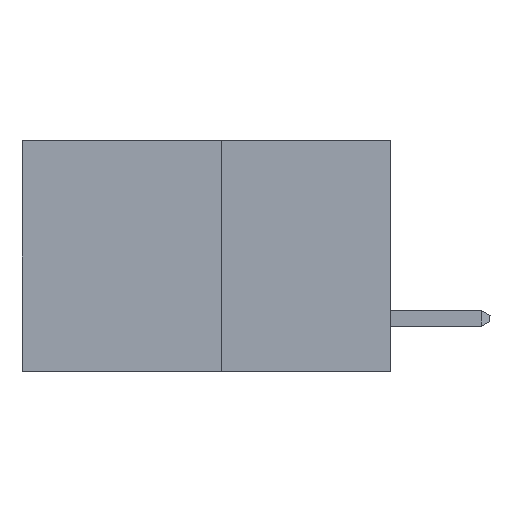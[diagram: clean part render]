
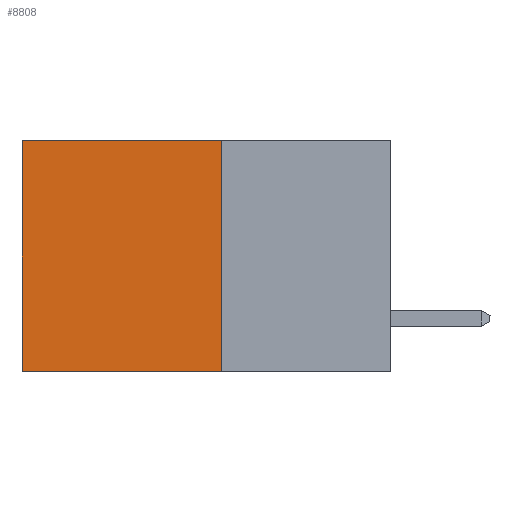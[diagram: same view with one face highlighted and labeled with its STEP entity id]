
A CAD part, left-side view. The second image highlights one B-rep face of the part: STEP entity #8808.
In plain terms, the highlighted planar face has unit normal (-1, 0, 0).
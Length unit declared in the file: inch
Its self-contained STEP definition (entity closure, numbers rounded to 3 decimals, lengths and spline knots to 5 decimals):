
#625 = VERTEX_POINT ( 'NONE', #13277 ) ;
#652 = EDGE_LOOP ( 'NONE', ( #5169, #15168, #2578, #5939 ) ) ;
#1002 = CARTESIAN_POINT ( 'NONE',  ( 0.277, 0.59, 0. ) ) ;
#1763 = CARTESIAN_POINT ( 'NONE',  ( 0.277, 0.27, -0.37 ) ) ;
#1943 = VERTEX_POINT ( 'NONE', #8669 ) ;
#2157 = EDGE_CURVE ( 'NONE', #6967, #1943, #5131, .T. ) ;
#2578 = ORIENTED_EDGE ( 'NONE', *, *, #9826, .F. ) ;
#4284 = LINE ( 'NONE', #13473, #10520 ) ;
#4394 = EDGE_CURVE ( 'NONE', #625, #14822, #4284, .T. ) ;
#4422 = DIRECTION ( 'NONE',  ( 0., 0., -1. ) ) ;
#4571 = CARTESIAN_POINT ( 'NONE',  ( 0.277, 0.27, -0.37 ) ) ;
#4724 = DIRECTION ( 'NONE',  ( 0., 1., 0. ) ) ;
#5131 = LINE ( 'NONE', #4571, #8038 ) ;
#5169 = ORIENTED_EDGE ( 'NONE', *, *, #15802, .T. ) ;
#5717 = AXIS2_PLACEMENT_3D ( 'NONE', #1763, #11905, #4422 ) ;
#5939 = ORIENTED_EDGE ( 'NONE', *, *, #4394, .T. ) ;
#6065 = CARTESIAN_POINT ( 'NONE',  ( 0.277, 0.27, -0.37 ) ) ;
#6291 = VECTOR ( 'NONE', #14464, 39.37008 ) ;
#6875 = CARTESIAN_POINT ( 'NONE',  ( 0.277, 0.27, -0.37 ) ) ;
#6967 = VERTEX_POINT ( 'NONE', #6065 ) ;
#7562 = FACE_OUTER_BOUND ( 'NONE', #652, .T. ) ;
#8038 = VECTOR ( 'NONE', #4724, 39.37008 ) ;
#8131 = DIRECTION ( 'NONE',  ( 0., 0., -1. ) ) ;
#8669 = CARTESIAN_POINT ( 'NONE',  ( 0.277, 0.59, -0.37 ) ) ;
#8808 = ADVANCED_FACE ( 'NONE', ( #7562 ), #10620, .F. ) ;
#9826 = EDGE_CURVE ( 'NONE', #625, #6967, #10088, .T. ) ;
#10088 = LINE ( 'NONE', #6875, #13067 ) ;
#10520 = VECTOR ( 'NONE', #13923, 39.37008 ) ;
#10620 = PLANE ( 'NONE',  #5717 ) ;
#11905 = DIRECTION ( 'NONE',  ( 1., 0., 0. ) ) ;
#13012 = LINE ( 'NONE', #13197, #6291 ) ;
#13067 = VECTOR ( 'NONE', #8131, 39.37008 ) ;
#13197 = CARTESIAN_POINT ( 'NONE',  ( 0.277, 0.59, -0.37 ) ) ;
#13277 = CARTESIAN_POINT ( 'NONE',  ( 0.277, 0.27, 0. ) ) ;
#13473 = CARTESIAN_POINT ( 'NONE',  ( 0.277, 0.27, 0. ) ) ;
#13923 = DIRECTION ( 'NONE',  ( 0., 1., 0. ) ) ;
#14464 = DIRECTION ( 'NONE',  ( 0., 0., -1. ) ) ;
#14822 = VERTEX_POINT ( 'NONE', #1002 ) ;
#15168 = ORIENTED_EDGE ( 'NONE', *, *, #2157, .F. ) ;
#15802 = EDGE_CURVE ( 'NONE', #14822, #1943, #13012, .T. ) ;
